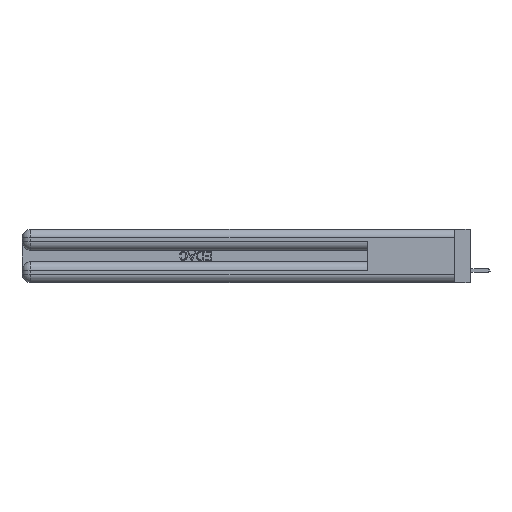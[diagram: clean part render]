
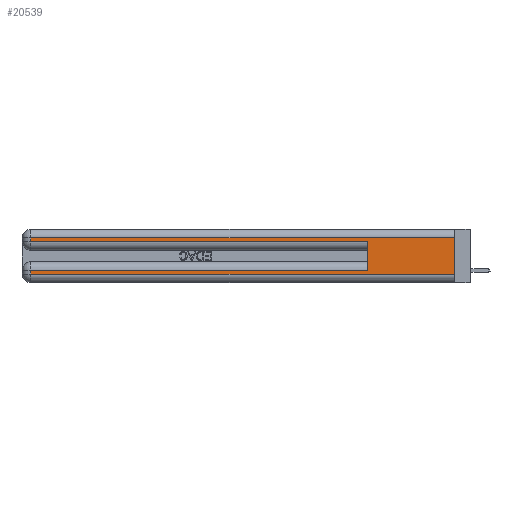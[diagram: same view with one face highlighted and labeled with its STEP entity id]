
A CAD part, left-side view. The second image highlights one B-rep face of the part: STEP entity #20539.
In plain terms, the highlighted planar face has unit normal (-1, 0, 0).
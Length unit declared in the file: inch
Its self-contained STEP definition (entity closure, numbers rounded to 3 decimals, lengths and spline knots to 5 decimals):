
#1487 = VECTOR ( 'NONE', #21179, 39.37008 ) ;
#1959 = CARTESIAN_POINT ( 'NONE',  ( 0., 0., 0.285 ) ) ;
#4140 = VECTOR ( 'NONE', #37644, 39.37008 ) ;
#5647 = DIRECTION ( 'NONE',  ( 1., 0., 0. ) ) ;
#6015 = AXIS2_PLACEMENT_3D ( 'NONE', #11828, #5647, #11413 ) ;
#6601 = EDGE_CURVE ( 'NONE', #32053, #31081, #40480, .T. ) ;
#8378 = DIRECTION ( 'NONE',  ( 0., -1., 0. ) ) ;
#8767 = VECTOR ( 'NONE', #17715, 39.37008 ) ;
#10014 = LINE ( 'NONE', #22754, #34106 ) ;
#10971 = CARTESIAN_POINT ( 'NONE',  ( 0., 0., 0.06 ) ) ;
#11038 = VERTEX_POINT ( 'NONE', #35012 ) ;
#11303 = VERTEX_POINT ( 'NONE', #10971 ) ;
#11413 = DIRECTION ( 'NONE',  ( 0., 0., -1. ) ) ;
#11828 = CARTESIAN_POINT ( 'NONE',  ( 0., 0., 0.37 ) ) ;
#12674 = ORIENTED_EDGE ( 'NONE', *, *, #18672, .T. ) ;
#13074 = VECTOR ( 'NONE', #22428, 39.37008 ) ;
#15036 = VECTOR ( 'NONE', #35300, 39.37008 ) ;
#16688 = EDGE_CURVE ( 'NONE', #39137, #11303, #28347, .T. ) ;
#17715 = DIRECTION ( 'NONE',  ( 0., -1., 0. ) ) ;
#17832 = CARTESIAN_POINT ( 'NONE',  ( 0., 2.94, 0.285 ) ) ;
#18623 = CARTESIAN_POINT ( 'NONE',  ( 0., 0., 0.37 ) ) ;
#18672 = EDGE_CURVE ( 'NONE', #38074, #39137, #19021, .T. ) ;
#19021 = LINE ( 'NONE', #40096, #1487 ) ;
#19829 = EDGE_CURVE ( 'NONE', #38707, #11038, #36690, .T. ) ;
#20494 = EDGE_CURVE ( 'NONE', #30603, #31081, #37119, .T. ) ;
#20539 = ADVANCED_FACE ( 'NONE', ( #33704 ), #39693, .F. ) ;
#21179 = DIRECTION ( 'NONE',  ( 0., 0., -1. ) ) ;
#21546 = CARTESIAN_POINT ( 'NONE',  ( 0., 2.94, 0.085 ) ) ;
#21655 = EDGE_CURVE ( 'NONE', #30603, #38074, #10014, .T. ) ;
#22428 = DIRECTION ( 'NONE',  ( 0., 0., 1. ) ) ;
#22754 = CARTESIAN_POINT ( 'NONE',  ( 0., 0., 0.085 ) ) ;
#23510 = ORIENTED_EDGE ( 'NONE', *, *, #16688, .T. ) ;
#23876 = CARTESIAN_POINT ( 'NONE',  ( 0., 0.6, 0.085 ) ) ;
#25526 = LINE ( 'NONE', #32266, #40338 ) ;
#27269 = ORIENTED_EDGE ( 'NONE', *, *, #32602, .T. ) ;
#27337 = CARTESIAN_POINT ( 'NONE',  ( 0., 0., 0.06 ) ) ;
#28347 = LINE ( 'NONE', #27337, #8767 ) ;
#28810 = CARTESIAN_POINT ( 'NONE',  ( 0., 0., 0.31 ) ) ;
#29215 = DIRECTION ( 'NONE',  ( 0., 0., -1. ) ) ;
#30603 = VERTEX_POINT ( 'NONE', #23876 ) ;
#31018 = EDGE_CURVE ( 'NONE', #38707, #11303, #40484, .T. ) ;
#31081 = VERTEX_POINT ( 'NONE', #38582 ) ;
#31299 = CARTESIAN_POINT ( 'NONE',  ( 0., 0., 0.31 ) ) ;
#31344 = EDGE_LOOP ( 'NONE', ( #32070, #38847, #27269, #32938, #32246, #40326, #12674, #23510 ) ) ;
#32053 = VERTEX_POINT ( 'NONE', #17832 ) ;
#32070 = ORIENTED_EDGE ( 'NONE', *, *, #31018, .F. ) ;
#32246 = ORIENTED_EDGE ( 'NONE', *, *, #20494, .F. ) ;
#32266 = CARTESIAN_POINT ( 'NONE',  ( 0., 2.94, 0.37 ) ) ;
#32598 = VECTOR ( 'NONE', #8378, 39.37008 ) ;
#32602 = EDGE_CURVE ( 'NONE', #11038, #32053, #25526, .T. ) ;
#32938 = ORIENTED_EDGE ( 'NONE', *, *, #6601, .T. ) ;
#33704 = FACE_OUTER_BOUND ( 'NONE', #31344, .T. ) ;
#34106 = VECTOR ( 'NONE', #38244, 39.37008 ) ;
#35012 = CARTESIAN_POINT ( 'NONE',  ( 0., 2.94, 0.31 ) ) ;
#35028 = CARTESIAN_POINT ( 'NONE',  ( 0., 0.6, 0.145 ) ) ;
#35300 = DIRECTION ( 'NONE',  ( 0., 1., 0. ) ) ;
#36384 = CARTESIAN_POINT ( 'NONE',  ( 0., 2.94, 0.06 ) ) ;
#36690 = LINE ( 'NONE', #28810, #15036 ) ;
#37119 = LINE ( 'NONE', #35028, #13074 ) ;
#37644 = DIRECTION ( 'NONE',  ( 0., 0., -1. ) ) ;
#38074 = VERTEX_POINT ( 'NONE', #21546 ) ;
#38244 = DIRECTION ( 'NONE',  ( 0., 1., 0. ) ) ;
#38582 = CARTESIAN_POINT ( 'NONE',  ( 0., 0.6, 0.285 ) ) ;
#38707 = VERTEX_POINT ( 'NONE', #31299 ) ;
#38847 = ORIENTED_EDGE ( 'NONE', *, *, #19829, .T. ) ;
#39137 = VERTEX_POINT ( 'NONE', #36384 ) ;
#39693 = PLANE ( 'NONE',  #6015 ) ;
#40096 = CARTESIAN_POINT ( 'NONE',  ( 0., 2.94, 0.37 ) ) ;
#40326 = ORIENTED_EDGE ( 'NONE', *, *, #21655, .T. ) ;
#40338 = VECTOR ( 'NONE', #29215, 39.37008 ) ;
#40480 = LINE ( 'NONE', #1959, #32598 ) ;
#40484 = LINE ( 'NONE', #18623, #4140 ) ;
